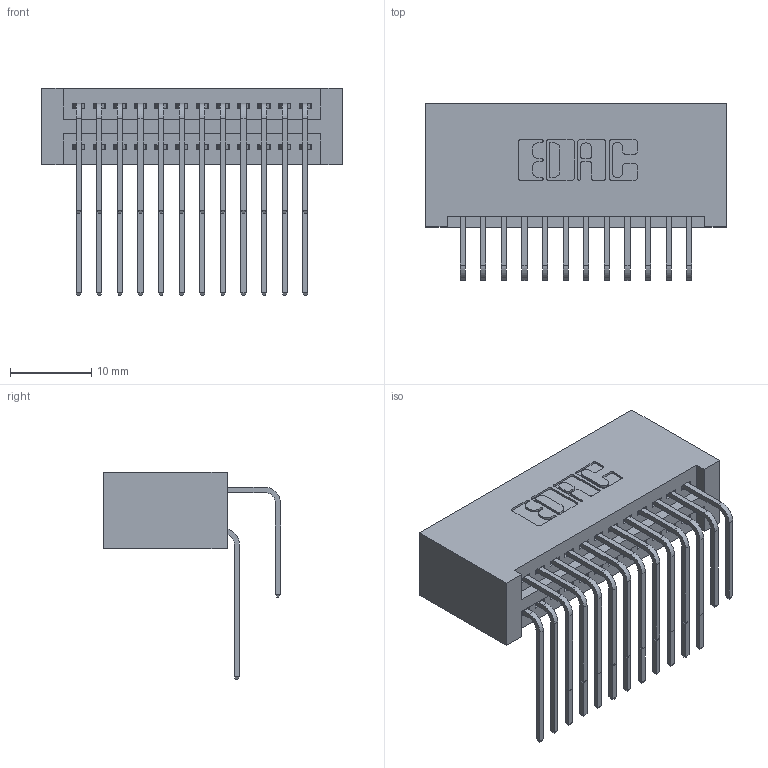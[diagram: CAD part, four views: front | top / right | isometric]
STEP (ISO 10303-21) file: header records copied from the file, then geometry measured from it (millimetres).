
FILE_DESCRIPTION (( 'STEP AP203' ), '1' );
FILE_NAME ('395-024-558-201.STEP', '2019-10-16T16:53:33', ( '' ), ( '' ), 'SwSTEP 2.0', 'SolidWorks 2016', '' );
FILE_SCHEMA (( 'CONFIG_CONTROL_DESIGN' ));
Length unit declared in the file: inch
Products named in the file (4): 345 Part_No Mounting Lugs; 345-292-001_558 559 Tail - 1; 345-292-001_558 Tail - 2; 395-024-558-201
Assembly tree (25 placements, depth 2):
  395-024-558-201
    345 Part_No Mounting Lugs
    345-292-001_558 559 Tail - 1  x12
    345-292-001_558 Tail - 2  x12
Bounding box: 37.08 x 21.83 x 25.53 mm (x, y, z)
Volume: 4078.3 mm3; surface area: 6401.6 mm2
Topology: 25 solids, 25 shells, 1366 faces, 4037 edges, 2658 vertices
Faces by surface type: plane 916, cylinder 450
Entity records: 14829 total; most frequent: CARTESIAN_POINT 2559, ORIENTED_EDGE 2442, DIRECTION 2261, EDGE_CURVE 1221, LINE 1009, VECTOR 1009, VERTEX_POINT 810, AXIS2_PLACEMENT_3D 626
